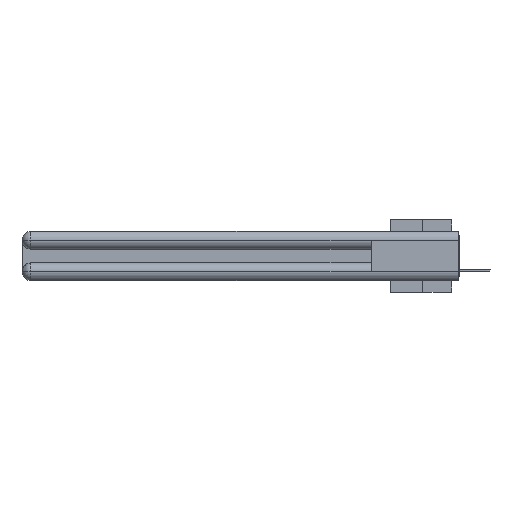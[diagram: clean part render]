
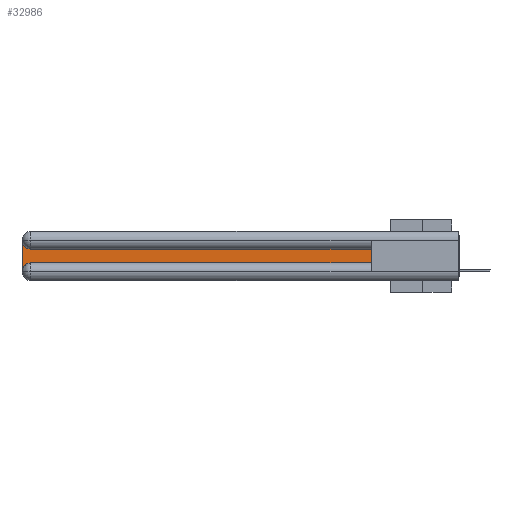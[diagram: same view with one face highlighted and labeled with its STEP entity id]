
A CAD part, left-side view. The second image highlights one B-rep face of the part: STEP entity #32986.
In plain terms, the highlighted planar face has unit normal (-1, 0, 0).
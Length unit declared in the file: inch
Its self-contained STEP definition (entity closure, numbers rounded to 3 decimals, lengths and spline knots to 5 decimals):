
#85 = AXIS2_PLACEMENT_3D ( 'NONE', #5882, #25321, #28696 ) ;
#705 = EDGE_CURVE ( 'NONE', #22282, #32211, #3795, .T. ) ;
#935 = DIRECTION ( 'NONE',  ( 0., 0., -1. ) ) ;
#2224 = EDGE_CURVE ( 'NONE', #32211, #21428, #4991, .T. ) ;
#2947 = ORIENTED_EDGE ( 'NONE', *, *, #705, .T. ) ;
#3152 = CARTESIAN_POINT ( 'NONE',  ( 0.075, 3., -0.1225 ) ) ;
#3782 = ORIENTED_EDGE ( 'NONE', *, *, #21959, .T. ) ;
#3795 = CIRCLE ( 'NONE', #21551, 0.06 ) ;
#4957 = CARTESIAN_POINT ( 'NONE',  ( 0.075, 2.94, -0.2175 ) ) ;
#4991 = LINE ( 'NONE', #12797, #19523 ) ;
#5477 = DIRECTION ( 'NONE',  ( 0., 0., -1. ) ) ;
#5882 = CARTESIAN_POINT ( 'NONE',  ( 0.075, 2.94, -0.0625 ) ) ;
#6473 = DIRECTION ( 'NONE',  ( 1., 0., 0. ) ) ;
#8681 = DIRECTION ( 'NONE',  ( 1., 0., 0. ) ) ;
#9579 = CARTESIAN_POINT ( 'NONE',  ( 0.075, 0.6, -0.2175 ) ) ;
#9688 = ORIENTED_EDGE ( 'NONE', *, *, #13787, .T. ) ;
#9968 = CARTESIAN_POINT ( 'NONE',  ( 0.075, 0.6, -0.1225 ) ) ;
#10467 = DIRECTION ( 'NONE',  ( 0., 0., 1. ) ) ;
#10505 = EDGE_CURVE ( 'NONE', #21428, #10900, #22722, .T. ) ;
#10874 = AXIS2_PLACEMENT_3D ( 'NONE', #3152, #8681, #31182 ) ;
#10900 = VERTEX_POINT ( 'NONE', #9968 ) ;
#12297 = VERTEX_POINT ( 'NONE', #21082 ) ;
#12511 = ORIENTED_EDGE ( 'NONE', *, *, #33523, .T. ) ;
#12797 = CARTESIAN_POINT ( 'NONE',  ( 0.075, 0.6, -0.2175 ) ) ;
#13787 = EDGE_CURVE ( 'NONE', #10900, #31443, #16057, .T. ) ;
#13823 = CARTESIAN_POINT ( 'NONE',  ( 0.075, 3., -0.2175 ) ) ;
#14059 = CIRCLE ( 'NONE', #85, 0.06 ) ;
#16010 = CARTESIAN_POINT ( 'NONE',  ( 0.075, 0.6, -0.2175 ) ) ;
#16057 = LINE ( 'NONE', #31500, #34456 ) ;
#17020 = VECTOR ( 'NONE', #10467, 39.37008 ) ;
#19523 = VECTOR ( 'NONE', #32463, 39.37008 ) ;
#19992 = PLANE ( 'NONE',  #10874 ) ;
#20107 = EDGE_LOOP ( 'NONE', ( #9688, #3782, #12511, #2947, #27356, #21545 ) ) ;
#21082 = CARTESIAN_POINT ( 'NONE',  ( 0.075, 3., -0.0625 ) ) ;
#21428 = VERTEX_POINT ( 'NONE', #9579 ) ;
#21545 = ORIENTED_EDGE ( 'NONE', *, *, #10505, .T. ) ;
#21551 = AXIS2_PLACEMENT_3D ( 'NONE', #34594, #6473, #935 ) ;
#21959 = EDGE_CURVE ( 'NONE', #31443, #12297, #14059, .T. ) ;
#22282 = VERTEX_POINT ( 'NONE', #28824 ) ;
#22722 = LINE ( 'NONE', #16010, #17020 ) ;
#23150 = DIRECTION ( 'NONE',  ( 0., 1., 0. ) ) ;
#25321 = DIRECTION ( 'NONE',  ( 1., 0., 0. ) ) ;
#27356 = ORIENTED_EDGE ( 'NONE', *, *, #2224, .T. ) ;
#27652 = FACE_OUTER_BOUND ( 'NONE', #20107, .T. ) ;
#28696 = DIRECTION ( 'NONE',  ( 0., 0., -1. ) ) ;
#28824 = CARTESIAN_POINT ( 'NONE',  ( 0.075, 3., -0.2775 ) ) ;
#29338 = CARTESIAN_POINT ( 'NONE',  ( 0.075, 2.94, -0.1225 ) ) ;
#31182 = DIRECTION ( 'NONE',  ( 0., 0., -1. ) ) ;
#31443 = VERTEX_POINT ( 'NONE', #29338 ) ;
#31500 = CARTESIAN_POINT ( 'NONE',  ( 0.075, 0.6, -0.1225 ) ) ;
#32211 = VERTEX_POINT ( 'NONE', #4957 ) ;
#32463 = DIRECTION ( 'NONE',  ( 0., -1., 0. ) ) ;
#32986 = ADVANCED_FACE ( 'NONE', ( #27652 ), #19992, .F. ) ;
#33523 = EDGE_CURVE ( 'NONE', #12297, #22282, #35498, .T. ) ;
#34456 = VECTOR ( 'NONE', #23150, 39.37008 ) ;
#34594 = CARTESIAN_POINT ( 'NONE',  ( 0.075, 2.94, -0.2775 ) ) ;
#35498 = LINE ( 'NONE', #13823, #36392 ) ;
#36392 = VECTOR ( 'NONE', #5477, 39.37008 ) ;
